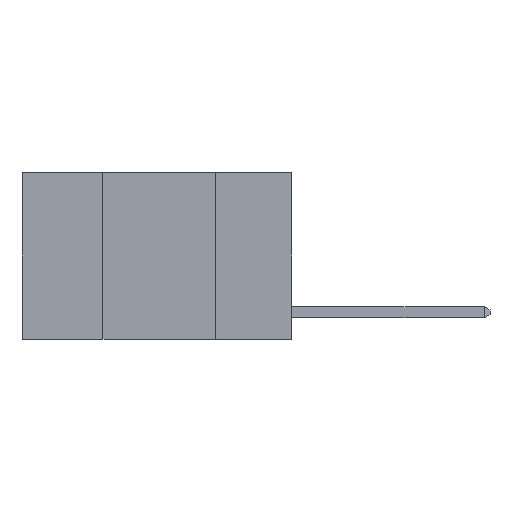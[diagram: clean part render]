
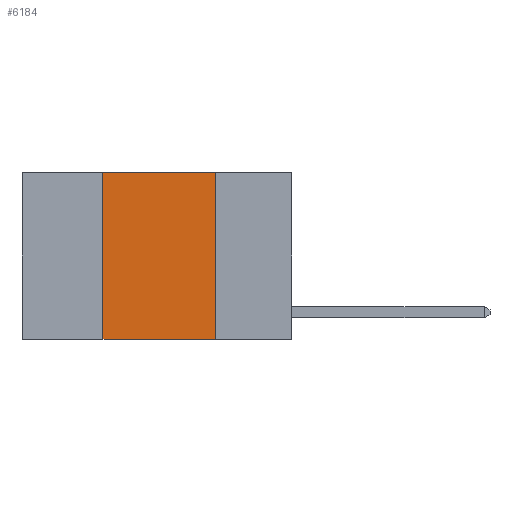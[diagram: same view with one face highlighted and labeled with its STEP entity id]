
A CAD part, left-side view. The second image highlights one B-rep face of the part: STEP entity #6184.
In plain terms, the highlighted planar face has unit normal (-1, 0, 0).
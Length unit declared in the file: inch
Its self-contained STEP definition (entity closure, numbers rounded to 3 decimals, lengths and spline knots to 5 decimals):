
#519 = VERTEX_POINT ( 'NONE', #6928 ) ;
#1227 = VECTOR ( 'NONE', #1369, 39.37008 ) ;
#1278 = VERTEX_POINT ( 'NONE', #4019 ) ;
#1369 = DIRECTION ( 'NONE',  ( 0., -1., 0. ) ) ;
#1531 = VECTOR ( 'NONE', #9670, 39.37008 ) ;
#1558 = VERTEX_POINT ( 'NONE', #8441 ) ;
#1707 = LINE ( 'NONE', #9922, #1531 ) ;
#2434 = VECTOR ( 'NONE', #7937, 39.37008 ) ;
#2580 = LINE ( 'NONE', #3700, #2434 ) ;
#2632 = EDGE_CURVE ( 'NONE', #6923, #519, #1707, .T. ) ;
#2673 = ORIENTED_EDGE ( 'NONE', *, *, #4375, .F. ) ;
#3246 = ORIENTED_EDGE ( 'NONE', *, *, #6062, .T. ) ;
#3386 = LINE ( 'NONE', #6930, #1227 ) ;
#3700 = CARTESIAN_POINT ( 'NONE',  ( 0., 0.17, 0. ) ) ;
#4019 = CARTESIAN_POINT ( 'NONE',  ( 0., 0.42, -0.37 ) ) ;
#4372 = EDGE_LOOP ( 'NONE', ( #2673, #5976, #4497, #3246 ) ) ;
#4375 = EDGE_CURVE ( 'NONE', #519, #1558, #2580, .T. ) ;
#4497 = ORIENTED_EDGE ( 'NONE', *, *, #4741, .F. ) ;
#4710 = VECTOR ( 'NONE', #8781, 39.37008 ) ;
#4741 = EDGE_CURVE ( 'NONE', #1278, #6923, #5596, .T. ) ;
#5596 = LINE ( 'NONE', #9058, #4710 ) ;
#5976 = ORIENTED_EDGE ( 'NONE', *, *, #2632, .F. ) ;
#6062 = EDGE_CURVE ( 'NONE', #1278, #1558, #3386, .T. ) ;
#6184 = ADVANCED_FACE ( 'NONE', ( #6592 ), #8963, .F. ) ;
#6384 = CARTESIAN_POINT ( 'NONE',  ( 0., 0.42, 0. ) ) ;
#6592 = FACE_OUTER_BOUND ( 'NONE', #4372, .T. ) ;
#6923 = VERTEX_POINT ( 'NONE', #6384 ) ;
#6928 = CARTESIAN_POINT ( 'NONE',  ( 0., 0.17, 0. ) ) ;
#6930 = CARTESIAN_POINT ( 'NONE',  ( 0., 0.6, -0.37 ) ) ;
#7937 = DIRECTION ( 'NONE',  ( 0., 0., -1. ) ) ;
#8441 = CARTESIAN_POINT ( 'NONE',  ( 0., 0.17, -0.37 ) ) ;
#8781 = DIRECTION ( 'NONE',  ( 0., 0., 1. ) ) ;
#8843 = DIRECTION ( 'NONE',  ( 0., 0., -1. ) ) ;
#8952 = DIRECTION ( 'NONE',  ( 1., 0., 0. ) ) ;
#8963 = PLANE ( 'NONE',  #9090 ) ;
#9058 = CARTESIAN_POINT ( 'NONE',  ( 0., 0.42, 0. ) ) ;
#9090 = AXIS2_PLACEMENT_3D ( 'NONE', #9505, #8952, #8843 ) ;
#9505 = CARTESIAN_POINT ( 'NONE',  ( 0., 0.6, 0. ) ) ;
#9670 = DIRECTION ( 'NONE',  ( 0., -1., 0. ) ) ;
#9922 = CARTESIAN_POINT ( 'NONE',  ( 0., 0.6, 0. ) ) ;
